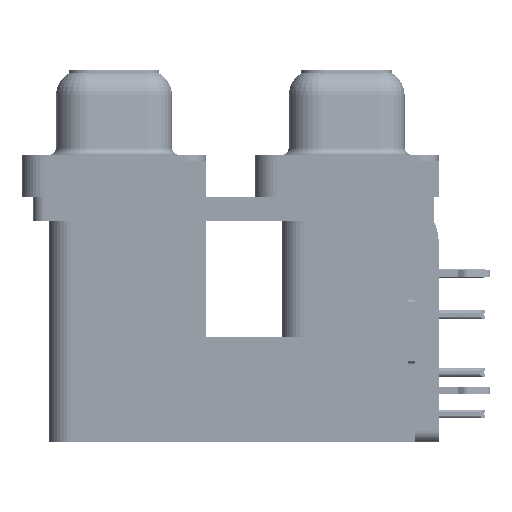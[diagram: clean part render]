
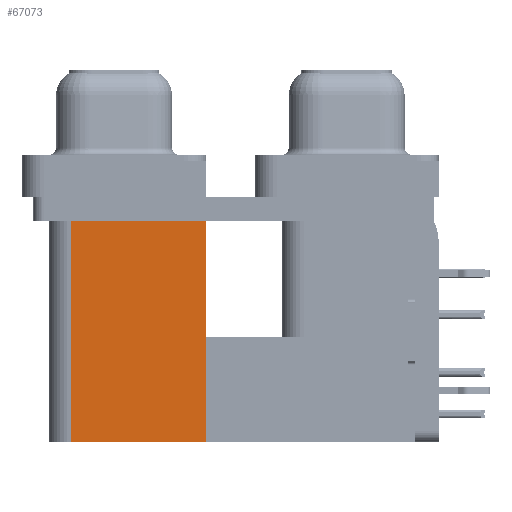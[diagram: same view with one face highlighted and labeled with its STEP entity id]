
A CAD part, left-side view. The second image highlights one B-rep face of the part: STEP entity #67073.
In plain terms, the highlighted planar face has unit normal (-1, 0, 0).
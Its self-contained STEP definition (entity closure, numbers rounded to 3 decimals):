
#2609 = LINE ( 'NONE', #74672, #53209 ) ;
#3392 = CARTESIAN_POINT ( 'NONE',  ( 3.79, 9.6, -19.2 ) ) ;
#3813 = LINE ( 'NONE', #27996, #60472 ) ;
#4559 = PLANE ( 'NONE',  #74523 ) ;
#6075 = CARTESIAN_POINT ( 'NONE',  ( 3.79, 9.6, -2.5 ) ) ;
#12751 = VERTEX_POINT ( 'NONE', #53778 ) ;
#14946 = VECTOR ( 'NONE', #52019, 1000. ) ;
#16448 = ORIENTED_EDGE ( 'NONE', *, *, #29777, .T. ) ;
#17144 = EDGE_CURVE ( 'NONE', #19479, #52213, #2609, .T. ) ;
#19479 = VERTEX_POINT ( 'NONE', #47605 ) ;
#19868 = EDGE_CURVE ( 'NONE', #52213, #12751, #47323, .T. ) ;
#22121 = DIRECTION ( 'NONE',  ( 1., 0., 0. ) ) ;
#23305 = DIRECTION ( 'NONE',  ( 0., 0., 1. ) ) ;
#27955 = CARTESIAN_POINT ( 'NONE',  ( 3.79, 9.6, -2.5 ) ) ;
#27996 = CARTESIAN_POINT ( 'NONE',  ( 3.79, 9.6, -19.2 ) ) ;
#28717 = DIRECTION ( 'NONE',  ( 0., 1., 0. ) ) ;
#29407 = CARTESIAN_POINT ( 'NONE',  ( 3.79, 18.8, -19.2 ) ) ;
#29777 = EDGE_CURVE ( 'NONE', #19479, #62404, #3813, .T. ) ;
#32431 = EDGE_LOOP ( 'NONE', ( #55519, #38310, #63044, #16448 ) ) ;
#37254 = EDGE_CURVE ( 'NONE', #62404, #12751, #45474, .T. ) ;
#38310 = ORIENTED_EDGE ( 'NONE', *, *, #19868, .F. ) ;
#38457 = DIRECTION ( 'NONE',  ( 0., 1., 0. ) ) ;
#45474 = LINE ( 'NONE', #27955, #73566 ) ;
#47323 = LINE ( 'NONE', #29407, #14946 ) ;
#47605 = CARTESIAN_POINT ( 'NONE',  ( 3.79, 9.6, -19.2 ) ) ;
#52019 = DIRECTION ( 'NONE',  ( 0., 0., 1. ) ) ;
#52213 = VERTEX_POINT ( 'NONE', #62047 ) ;
#53209 = VECTOR ( 'NONE', #38457, 1000. ) ;
#53778 = CARTESIAN_POINT ( 'NONE',  ( 3.79, 18.8, -2.5 ) ) ;
#55519 = ORIENTED_EDGE ( 'NONE', *, *, #37254, .T. ) ;
#60472 = VECTOR ( 'NONE', #23305, 1000. ) ;
#62047 = CARTESIAN_POINT ( 'NONE',  ( 3.79, 18.8, -19.2 ) ) ;
#62251 = FACE_OUTER_BOUND ( 'NONE', #32431, .T. ) ;
#62404 = VERTEX_POINT ( 'NONE', #6075 ) ;
#63044 = ORIENTED_EDGE ( 'NONE', *, *, #17144, .F. ) ;
#67073 = ADVANCED_FACE ( 'NONE', ( #62251 ), #4559, .F. ) ;
#68876 = DIRECTION ( 'NONE',  ( 0., 0., -1. ) ) ;
#73566 = VECTOR ( 'NONE', #28717, 1000. ) ;
#74523 = AXIS2_PLACEMENT_3D ( 'NONE', #3392, #22121, #68876 ) ;
#74672 = CARTESIAN_POINT ( 'NONE',  ( 3.79, 9.6, -19.2 ) ) ;
